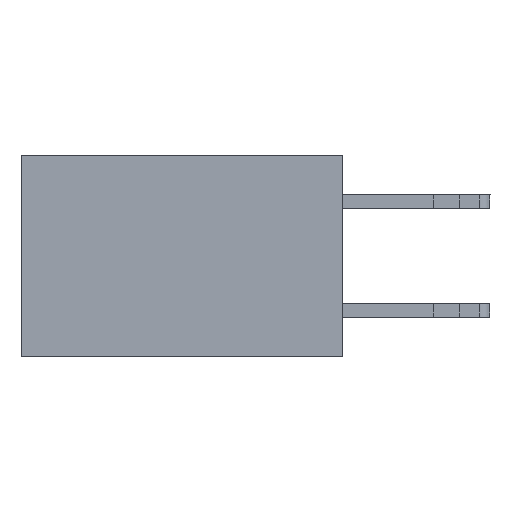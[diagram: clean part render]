
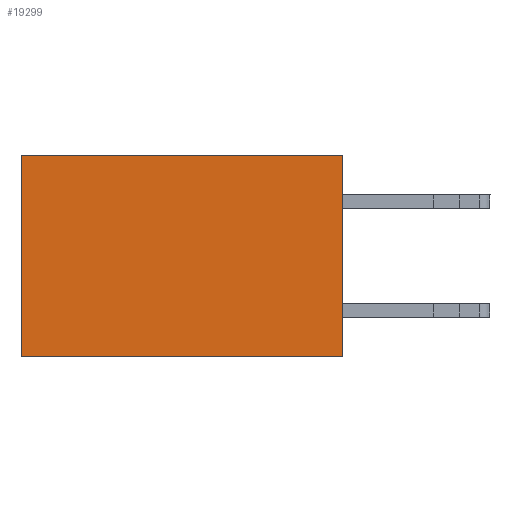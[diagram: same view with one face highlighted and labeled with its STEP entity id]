
A CAD part, left-side view. The second image highlights one B-rep face of the part: STEP entity #19299.
In plain terms, the highlighted planar face has unit normal (-1, 0, 0).
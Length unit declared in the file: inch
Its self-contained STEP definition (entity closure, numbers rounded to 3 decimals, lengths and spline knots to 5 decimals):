
#986 = CARTESIAN_POINT ( 'NONE',  ( 0.277, 0., -0.37 ) ) ;
#1704 = LINE ( 'NONE', #16640, #16042 ) ;
#2002 = ORIENTED_EDGE ( 'NONE', *, *, #4928, .F. ) ;
#2571 = CARTESIAN_POINT ( 'NONE',  ( 0.277, 0., -0.37 ) ) ;
#3606 = EDGE_LOOP ( 'NONE', ( #10464, #2002, #17773, #13120 ) ) ;
#4928 = EDGE_CURVE ( 'NONE', #6844, #10165, #8403, .T. ) ;
#5518 = VERTEX_POINT ( 'NONE', #21884 ) ;
#5687 = EDGE_CURVE ( 'NONE', #5518, #13248, #1704, .T. ) ;
#5715 = DIRECTION ( 'NONE',  ( 0., 1., 0. ) ) ;
#5955 = EDGE_CURVE ( 'NONE', #13248, #10165, #15661, .T. ) ;
#6708 = VECTOR ( 'NONE', #15439, 39.37008 ) ;
#6844 = VERTEX_POINT ( 'NONE', #21033 ) ;
#7792 = AXIS2_PLACEMENT_3D ( 'NONE', #14384, #17792, #21793 ) ;
#7861 = CARTESIAN_POINT ( 'NONE',  ( 0.277, 0.59, -0.37 ) ) ;
#8278 = LINE ( 'NONE', #986, #23102 ) ;
#8403 = LINE ( 'NONE', #2571, #6708 ) ;
#10165 = VERTEX_POINT ( 'NONE', #7861 ) ;
#10464 = ORIENTED_EDGE ( 'NONE', *, *, #5955, .T. ) ;
#13120 = ORIENTED_EDGE ( 'NONE', *, *, #5687, .T. ) ;
#13248 = VERTEX_POINT ( 'NONE', #17749 ) ;
#14384 = CARTESIAN_POINT ( 'NONE',  ( 0.277, 0., -0.37 ) ) ;
#14828 = EDGE_CURVE ( 'NONE', #5518, #6844, #8278, .T. ) ;
#15285 = CARTESIAN_POINT ( 'NONE',  ( 0.277, 0.59, -0.37 ) ) ;
#15439 = DIRECTION ( 'NONE',  ( 0., 1., 0. ) ) ;
#15661 = LINE ( 'NONE', #15285, #22656 ) ;
#15686 = DIRECTION ( 'NONE',  ( 0., 0., -1. ) ) ;
#16042 = VECTOR ( 'NONE', #5715, 39.37008 ) ;
#16640 = CARTESIAN_POINT ( 'NONE',  ( 0.277, 0., 0. ) ) ;
#17749 = CARTESIAN_POINT ( 'NONE',  ( 0.277, 0.59, 0. ) ) ;
#17773 = ORIENTED_EDGE ( 'NONE', *, *, #14828, .F. ) ;
#17792 = DIRECTION ( 'NONE',  ( 1., 0., 0. ) ) ;
#18147 = PLANE ( 'NONE',  #7792 ) ;
#19299 = ADVANCED_FACE ( 'NONE', ( #23627 ), #18147, .F. ) ;
#20880 = DIRECTION ( 'NONE',  ( 0., 0., -1. ) ) ;
#21033 = CARTESIAN_POINT ( 'NONE',  ( 0.277, 0., -0.37 ) ) ;
#21793 = DIRECTION ( 'NONE',  ( 0., 0., -1. ) ) ;
#21884 = CARTESIAN_POINT ( 'NONE',  ( 0.277, 0., 0. ) ) ;
#22656 = VECTOR ( 'NONE', #20880, 39.37008 ) ;
#23102 = VECTOR ( 'NONE', #15686, 39.37008 ) ;
#23627 = FACE_OUTER_BOUND ( 'NONE', #3606, .T. ) ;
